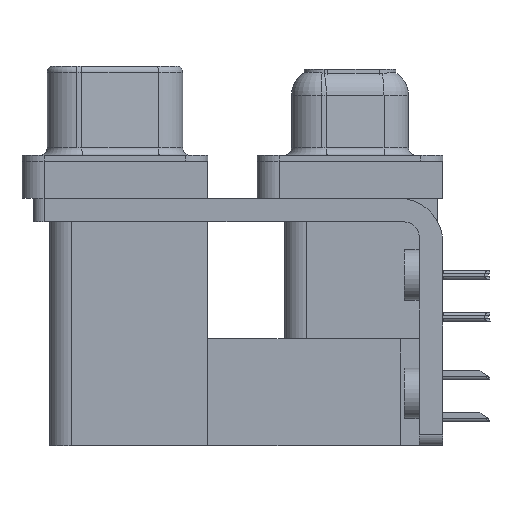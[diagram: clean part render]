
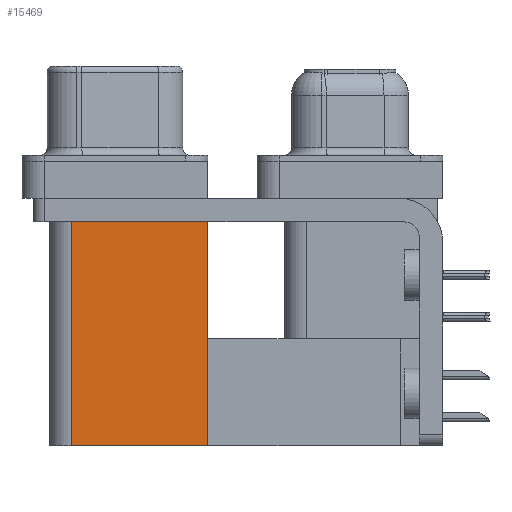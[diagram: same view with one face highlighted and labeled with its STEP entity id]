
A CAD part, left-side view. The second image highlights one B-rep face of the part: STEP entity #15469.
In plain terms, the highlighted planar face has unit normal (-1, 0, 0).
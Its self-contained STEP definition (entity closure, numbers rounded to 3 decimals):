
#650 = ORIENTED_EDGE ( 'NONE', *, *, #15159, .T. ) ;
#1036 = VECTOR ( 'NONE', #11280, 1000. ) ;
#3278 = DIRECTION ( 'NONE',  ( 1., 0., 0. ) ) ;
#3691 = FACE_OUTER_BOUND ( 'NONE', #29520, .T. ) ;
#4361 = VERTEX_POINT ( 'NONE', #27805 ) ;
#6940 = VECTOR ( 'NONE', #22260, 1000. ) ;
#8646 = CARTESIAN_POINT ( 'NONE',  ( 3.765, 9.6, -19.2 ) ) ;
#9759 = ORIENTED_EDGE ( 'NONE', *, *, #13573, .T. ) ;
#11019 = DIRECTION ( 'NONE',  ( 0., 0., -1. ) ) ;
#11280 = DIRECTION ( 'NONE',  ( 0., 1., 0. ) ) ;
#11498 = CARTESIAN_POINT ( 'NONE',  ( 3.765, 9.6, -19.2 ) ) ;
#11959 = CARTESIAN_POINT ( 'NONE',  ( 3.765, 9.6, -2.5 ) ) ;
#13573 = EDGE_CURVE ( 'NONE', #31019, #4361, #21591, .T. ) ;
#15159 = EDGE_CURVE ( 'NONE', #4361, #39913, #18192, .T. ) ;
#15290 = DIRECTION ( 'NONE',  ( 0., 1., 0. ) ) ;
#15469 = ADVANCED_FACE ( 'NONE', ( #3691 ), #40682, .F. ) ;
#18192 = LINE ( 'NONE', #11959, #1036 ) ;
#21591 = LINE ( 'NONE', #8646, #6940 ) ;
#22063 = CARTESIAN_POINT ( 'NONE',  ( 3.765, 18.8, -2.5 ) ) ;
#22260 = DIRECTION ( 'NONE',  ( 0., 0., 1. ) ) ;
#23324 = CARTESIAN_POINT ( 'NONE',  ( 3.765, 9.6, -19.2 ) ) ;
#24884 = LINE ( 'NONE', #11498, #30401 ) ;
#26627 = CARTESIAN_POINT ( 'NONE',  ( 3.765, 18.8, -19.2 ) ) ;
#27805 = CARTESIAN_POINT ( 'NONE',  ( 3.765, 9.6, -2.5 ) ) ;
#28231 = CARTESIAN_POINT ( 'NONE',  ( 3.765, 18.8, -19.2 ) ) ;
#28278 = EDGE_CURVE ( 'NONE', #31019, #33232, #24884, .T. ) ;
#29520 = EDGE_LOOP ( 'NONE', ( #650, #40509, #38779, #9759 ) ) ;
#30401 = VECTOR ( 'NONE', #15290, 1000. ) ;
#31019 = VERTEX_POINT ( 'NONE', #23324 ) ;
#31330 = EDGE_CURVE ( 'NONE', #33232, #39913, #36441, .T. ) ;
#33232 = VERTEX_POINT ( 'NONE', #28231 ) ;
#34373 = VECTOR ( 'NONE', #36010, 1000. ) ;
#36010 = DIRECTION ( 'NONE',  ( 0., 0., 1. ) ) ;
#36441 = LINE ( 'NONE', #26627, #34373 ) ;
#38779 = ORIENTED_EDGE ( 'NONE', *, *, #28278, .F. ) ;
#39913 = VERTEX_POINT ( 'NONE', #22063 ) ;
#40509 = ORIENTED_EDGE ( 'NONE', *, *, #31330, .F. ) ;
#40682 = PLANE ( 'NONE',  #42740 ) ;
#41319 = CARTESIAN_POINT ( 'NONE',  ( 3.765, 9.6, -19.2 ) ) ;
#42740 = AXIS2_PLACEMENT_3D ( 'NONE', #41319, #3278, #11019 ) ;
